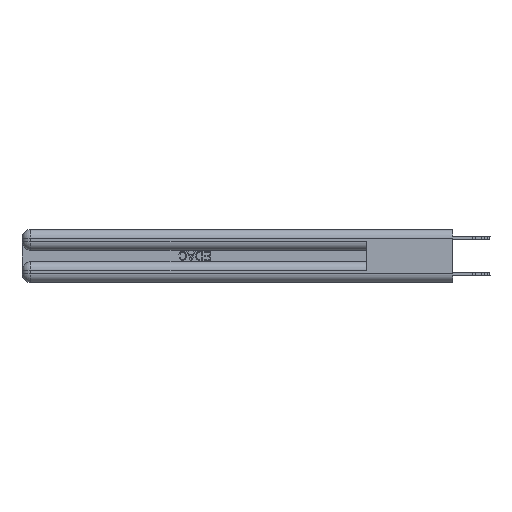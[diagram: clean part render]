
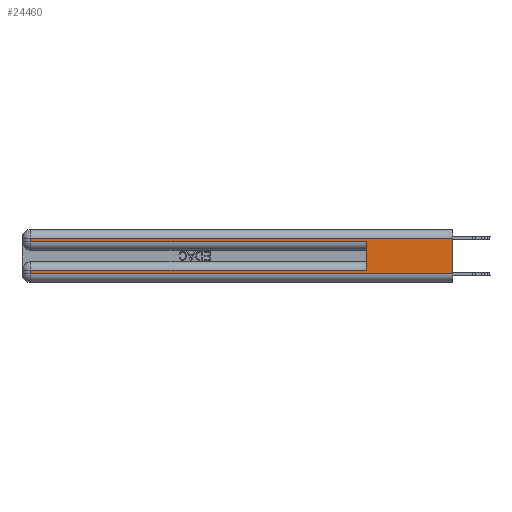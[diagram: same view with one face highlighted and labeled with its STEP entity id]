
A CAD part, left-side view. The second image highlights one B-rep face of the part: STEP entity #24460.
In plain terms, the highlighted planar face has unit normal (-1, 0, 0).
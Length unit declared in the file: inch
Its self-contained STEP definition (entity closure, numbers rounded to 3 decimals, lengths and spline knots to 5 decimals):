
#233 = LINE ( 'NONE', #29256, #17223 ) ;
#287 = DIRECTION ( 'NONE',  ( 0., 0., 1. ) ) ;
#1426 = ORIENTED_EDGE ( 'NONE', *, *, #1799, .T. ) ;
#1586 = VECTOR ( 'NONE', #7696, 39.37008 ) ;
#1695 = DIRECTION ( 'NONE',  ( 0., 1., 0. ) ) ;
#1799 = EDGE_CURVE ( 'NONE', #15440, #13148, #30979, .T. ) ;
#1931 = CARTESIAN_POINT ( 'NONE',  ( 0., 0., 0.285 ) ) ;
#3774 = AXIS2_PLACEMENT_3D ( 'NONE', #21790, #13234, #32649 ) ;
#4573 = CARTESIAN_POINT ( 'NONE',  ( 0., 0., 0.06 ) ) ;
#5013 = DIRECTION ( 'NONE',  ( 0., 1., 0. ) ) ;
#5340 = CARTESIAN_POINT ( 'NONE',  ( 0., 0.6, 0.145 ) ) ;
#5630 = EDGE_LOOP ( 'NONE', ( #33747, #25819, #30633, #1426, #25873, #29200, #25357, #18712 ) ) ;
#6161 = DIRECTION ( 'NONE',  ( 0., 0., -1. ) ) ;
#6348 = VECTOR ( 'NONE', #1695, 39.37008 ) ;
#7696 = DIRECTION ( 'NONE',  ( 0., 0., -1. ) ) ;
#8399 = EDGE_CURVE ( 'NONE', #12417, #15220, #31093, .T. ) ;
#8653 = EDGE_CURVE ( 'NONE', #32224, #13148, #29306, .T. ) ;
#9984 = CARTESIAN_POINT ( 'NONE',  ( 0., 2.94, 0.37 ) ) ;
#10151 = LINE ( 'NONE', #9984, #1586 ) ;
#12069 = CARTESIAN_POINT ( 'NONE',  ( 0., 0., 0.31 ) ) ;
#12417 = VERTEX_POINT ( 'NONE', #12069 ) ;
#13148 = VERTEX_POINT ( 'NONE', #17389 ) ;
#13234 = DIRECTION ( 'NONE',  ( 1., 0., 0. ) ) ;
#13759 = FACE_OUTER_BOUND ( 'NONE', #5630, .T. ) ;
#14343 = DIRECTION ( 'NONE',  ( 0., 0., -1. ) ) ;
#15220 = VERTEX_POINT ( 'NONE', #24481 ) ;
#15440 = VERTEX_POINT ( 'NONE', #23581 ) ;
#16190 = VECTOR ( 'NONE', #6161, 39.37008 ) ;
#17223 = VECTOR ( 'NONE', #29779, 39.37008 ) ;
#17389 = CARTESIAN_POINT ( 'NONE',  ( 0., 0.6, 0.285 ) ) ;
#17878 = CARTESIAN_POINT ( 'NONE',  ( 0., 2.94, 0.085 ) ) ;
#18152 = LINE ( 'NONE', #28973, #20617 ) ;
#18712 = ORIENTED_EDGE ( 'NONE', *, *, #26687, .T. ) ;
#19741 = VECTOR ( 'NONE', #287, 39.37008 ) ;
#19787 = CARTESIAN_POINT ( 'NONE',  ( 0., 2.94, 0.37 ) ) ;
#20582 = CARTESIAN_POINT ( 'NONE',  ( 0., 0., 0.31 ) ) ;
#20617 = VECTOR ( 'NONE', #5013, 39.37008 ) ;
#21067 = CARTESIAN_POINT ( 'NONE',  ( 0., 2.94, 0.06 ) ) ;
#21163 = CARTESIAN_POINT ( 'NONE',  ( 0., 0.6, 0.085 ) ) ;
#21790 = CARTESIAN_POINT ( 'NONE',  ( 0., 0., 0.37 ) ) ;
#22745 = LINE ( 'NONE', #19787, #16190 ) ;
#23244 = DIRECTION ( 'NONE',  ( 0., -1., 0. ) ) ;
#23581 = CARTESIAN_POINT ( 'NONE',  ( 0., 2.94, 0.285 ) ) ;
#24460 = ADVANCED_FACE ( 'NONE', ( #13759 ), #29328, .F. ) ;
#24481 = CARTESIAN_POINT ( 'NONE',  ( 0., 2.94, 0.31 ) ) ;
#25053 = VECTOR ( 'NONE', #23244, 39.37008 ) ;
#25357 = ORIENTED_EDGE ( 'NONE', *, *, #28338, .T. ) ;
#25819 = ORIENTED_EDGE ( 'NONE', *, *, #8399, .T. ) ;
#25873 = ORIENTED_EDGE ( 'NONE', *, *, #8653, .F. ) ;
#26687 = EDGE_CURVE ( 'NONE', #28823, #27112, #233, .T. ) ;
#27112 = VERTEX_POINT ( 'NONE', #4573 ) ;
#28003 = LINE ( 'NONE', #33073, #30244 ) ;
#28338 = EDGE_CURVE ( 'NONE', #32052, #28823, #22745, .T. ) ;
#28823 = VERTEX_POINT ( 'NONE', #21067 ) ;
#28973 = CARTESIAN_POINT ( 'NONE',  ( 0., 0., 0.085 ) ) ;
#29200 = ORIENTED_EDGE ( 'NONE', *, *, #33188, .T. ) ;
#29256 = CARTESIAN_POINT ( 'NONE',  ( 0., 0., 0.06 ) ) ;
#29306 = LINE ( 'NONE', #5340, #19741 ) ;
#29328 = PLANE ( 'NONE',  #3774 ) ;
#29779 = DIRECTION ( 'NONE',  ( 0., -1., 0. ) ) ;
#30244 = VECTOR ( 'NONE', #14343, 39.37008 ) ;
#30591 = EDGE_CURVE ( 'NONE', #12417, #27112, #28003, .T. ) ;
#30633 = ORIENTED_EDGE ( 'NONE', *, *, #32248, .T. ) ;
#30979 = LINE ( 'NONE', #1931, #25053 ) ;
#31093 = LINE ( 'NONE', #20582, #6348 ) ;
#32052 = VERTEX_POINT ( 'NONE', #17878 ) ;
#32224 = VERTEX_POINT ( 'NONE', #21163 ) ;
#32248 = EDGE_CURVE ( 'NONE', #15220, #15440, #10151, .T. ) ;
#32649 = DIRECTION ( 'NONE',  ( 0., 0., -1. ) ) ;
#33073 = CARTESIAN_POINT ( 'NONE',  ( 0., 0., 0.37 ) ) ;
#33188 = EDGE_CURVE ( 'NONE', #32224, #32052, #18152, .T. ) ;
#33747 = ORIENTED_EDGE ( 'NONE', *, *, #30591, .F. ) ;
